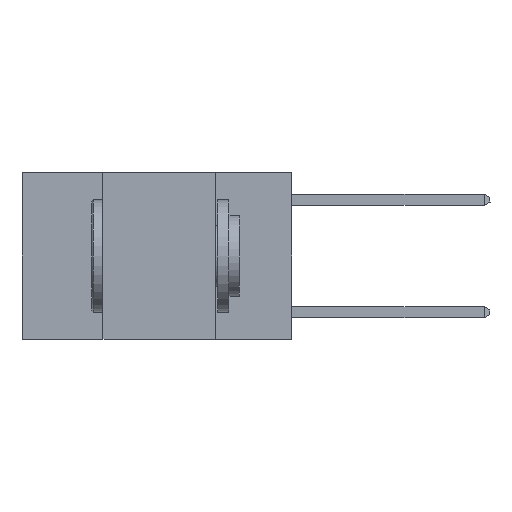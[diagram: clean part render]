
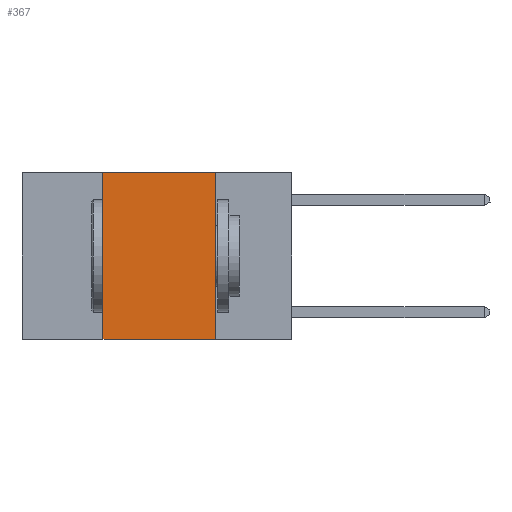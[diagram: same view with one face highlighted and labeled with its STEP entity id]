
A CAD part, left-side view. The second image highlights one B-rep face of the part: STEP entity #367.
In plain terms, the highlighted planar face has unit normal (-1, 0, 0).
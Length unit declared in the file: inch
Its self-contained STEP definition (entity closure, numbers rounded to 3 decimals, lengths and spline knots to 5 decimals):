
#367 = ADVANCED_FACE ( 'NONE', ( #3326 ), #6615, .F. ) ;
#397 = CARTESIAN_POINT ( 'NONE',  ( 0., 0.17, 0. ) ) ;
#875 = VERTEX_POINT ( 'NONE', #9876 ) ;
#1080 = CARTESIAN_POINT ( 'NONE',  ( 0., 0.6, -0.37 ) ) ;
#1770 = CARTESIAN_POINT ( 'NONE',  ( 0., 0.42, 0. ) ) ;
#1892 = CARTESIAN_POINT ( 'NONE',  ( 0., 0.6, 0. ) ) ;
#2592 = DIRECTION ( 'NONE',  ( 0., 0., -1. ) ) ;
#2808 = DIRECTION ( 'NONE',  ( 0., -1., 0. ) ) ;
#2990 = ORIENTED_EDGE ( 'NONE', *, *, #9243, .T. ) ;
#3326 = FACE_OUTER_BOUND ( 'NONE', #8857, .T. ) ;
#3586 = LINE ( 'NONE', #1080, #8308 ) ;
#3741 = VECTOR ( 'NONE', #8942, 39.37008 ) ;
#3865 = EDGE_CURVE ( 'NONE', #4871, #7565, #8454, .T. ) ;
#4871 = VERTEX_POINT ( 'NONE', #8157 ) ;
#6183 = EDGE_CURVE ( 'NONE', #6821, #875, #8963, .T. ) ;
#6195 = CARTESIAN_POINT ( 'NONE',  ( 0., 0.6, 0. ) ) ;
#6615 = PLANE ( 'NONE',  #9291 ) ;
#6620 = VECTOR ( 'NONE', #2592, 39.37008 ) ;
#6821 = VERTEX_POINT ( 'NONE', #397 ) ;
#7331 = VECTOR ( 'NONE', #2808, 39.37008 ) ;
#7565 = VERTEX_POINT ( 'NONE', #8648 ) ;
#7600 = LINE ( 'NONE', #1892, #7331 ) ;
#8058 = DIRECTION ( 'NONE',  ( 1., 0., 0. ) ) ;
#8157 = CARTESIAN_POINT ( 'NONE',  ( 0., 0.42, -0.37 ) ) ;
#8308 = VECTOR ( 'NONE', #8309, 39.37008 ) ;
#8309 = DIRECTION ( 'NONE',  ( 0., -1., 0. ) ) ;
#8454 = LINE ( 'NONE', #1770, #3741 ) ;
#8648 = CARTESIAN_POINT ( 'NONE',  ( 0., 0.42, 0. ) ) ;
#8838 = CARTESIAN_POINT ( 'NONE',  ( 0., 0.17, 0. ) ) ;
#8857 = EDGE_LOOP ( 'NONE', ( #11050, #10087, #9873, #2990 ) ) ;
#8942 = DIRECTION ( 'NONE',  ( 0., 0., 1. ) ) ;
#8963 = LINE ( 'NONE', #8838, #6620 ) ;
#9243 = EDGE_CURVE ( 'NONE', #4871, #875, #3586, .T. ) ;
#9291 = AXIS2_PLACEMENT_3D ( 'NONE', #6195, #8058, #11113 ) ;
#9873 = ORIENTED_EDGE ( 'NONE', *, *, #3865, .F. ) ;
#9876 = CARTESIAN_POINT ( 'NONE',  ( 0., 0.17, -0.37 ) ) ;
#10087 = ORIENTED_EDGE ( 'NONE', *, *, #11626, .F. ) ;
#11050 = ORIENTED_EDGE ( 'NONE', *, *, #6183, .F. ) ;
#11113 = DIRECTION ( 'NONE',  ( 0., 0., -1. ) ) ;
#11626 = EDGE_CURVE ( 'NONE', #7565, #6821, #7600, .T. ) ;
